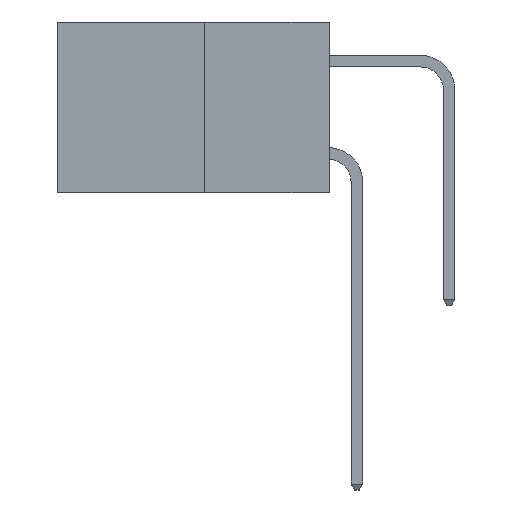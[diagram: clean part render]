
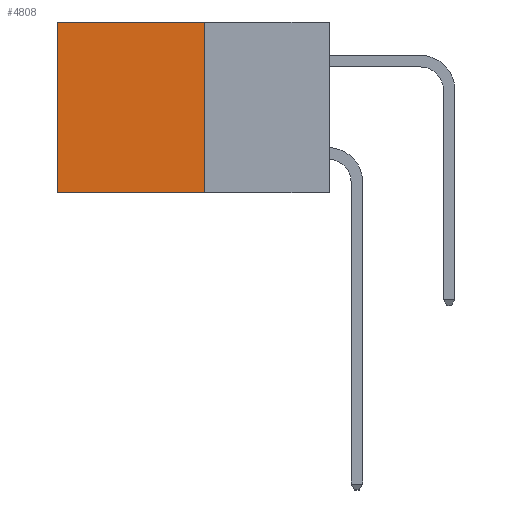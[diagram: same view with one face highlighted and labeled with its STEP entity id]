
A CAD part, left-side view. The second image highlights one B-rep face of the part: STEP entity #4808.
In plain terms, the highlighted planar face has unit normal (-1, 0, 0).
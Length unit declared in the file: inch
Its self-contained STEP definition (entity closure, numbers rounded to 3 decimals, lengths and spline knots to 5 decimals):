
#404 = VERTEX_POINT ( 'NONE', #9506 ) ;
#1566 = EDGE_LOOP ( 'NONE', ( #14040, #3874, #6951, #15306 ) ) ;
#2842 = CARTESIAN_POINT ( 'NONE',  ( 0.277, 0.27, 0. ) ) ;
#3370 = AXIS2_PLACEMENT_3D ( 'NONE', #3706, #5290, #5269 ) ;
#3593 = LINE ( 'NONE', #17458, #17728 ) ;
#3667 = CARTESIAN_POINT ( 'NONE',  ( 0.277, 0.59, 0. ) ) ;
#3706 = CARTESIAN_POINT ( 'NONE',  ( 0.277, 0.27, -0.37 ) ) ;
#3874 = ORIENTED_EDGE ( 'NONE', *, *, #10341, .F. ) ;
#4452 = EDGE_CURVE ( 'NONE', #16683, #404, #9356, .T. ) ;
#4583 = CARTESIAN_POINT ( 'NONE',  ( 0.277, 0.27, -0.37 ) ) ;
#4590 = VERTEX_POINT ( 'NONE', #4583 ) ;
#4808 = ADVANCED_FACE ( 'NONE', ( #14669 ), #5573, .F. ) ;
#5269 = DIRECTION ( 'NONE',  ( 0., 0., -1. ) ) ;
#5290 = DIRECTION ( 'NONE',  ( 1., 0., 0. ) ) ;
#5573 = PLANE ( 'NONE',  #3370 ) ;
#6177 = LINE ( 'NONE', #8013, #16674 ) ;
#6951 = ORIENTED_EDGE ( 'NONE', *, *, #8667, .F. ) ;
#7421 = DIRECTION ( 'NONE',  ( 0., 0., -1. ) ) ;
#8013 = CARTESIAN_POINT ( 'NONE',  ( 0.277, 0.27, -0.37 ) ) ;
#8667 = EDGE_CURVE ( 'NONE', #16615, #4590, #6177, .T. ) ;
#8853 = CARTESIAN_POINT ( 'NONE',  ( 0.277, 0.27, 0. ) ) ;
#9356 = LINE ( 'NONE', #9550, #16152 ) ;
#9506 = CARTESIAN_POINT ( 'NONE',  ( 0.277, 0.59, -0.37 ) ) ;
#9550 = CARTESIAN_POINT ( 'NONE',  ( 0.277, 0.59, -0.37 ) ) ;
#9570 = DIRECTION ( 'NONE',  ( 0., 0., -1. ) ) ;
#10341 = EDGE_CURVE ( 'NONE', #4590, #404, #3593, .T. ) ;
#10536 = VECTOR ( 'NONE', #11212, 39.37008 ) ;
#11212 = DIRECTION ( 'NONE',  ( 0., 1., 0. ) ) ;
#11925 = EDGE_CURVE ( 'NONE', #16615, #16683, #14161, .T. ) ;
#14040 = ORIENTED_EDGE ( 'NONE', *, *, #4452, .T. ) ;
#14161 = LINE ( 'NONE', #2842, #10536 ) ;
#14669 = FACE_OUTER_BOUND ( 'NONE', #1566, .T. ) ;
#14864 = DIRECTION ( 'NONE',  ( 0., 1., 0. ) ) ;
#15306 = ORIENTED_EDGE ( 'NONE', *, *, #11925, .T. ) ;
#16152 = VECTOR ( 'NONE', #9570, 39.37008 ) ;
#16615 = VERTEX_POINT ( 'NONE', #8853 ) ;
#16674 = VECTOR ( 'NONE', #7421, 39.37008 ) ;
#16683 = VERTEX_POINT ( 'NONE', #3667 ) ;
#17458 = CARTESIAN_POINT ( 'NONE',  ( 0.277, 0.27, -0.37 ) ) ;
#17728 = VECTOR ( 'NONE', #14864, 39.37008 ) ;
